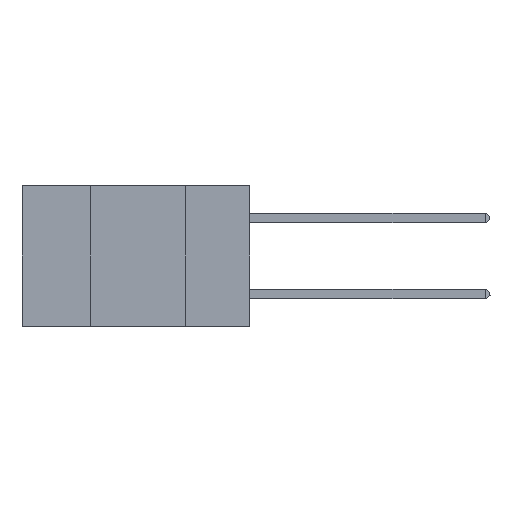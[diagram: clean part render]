
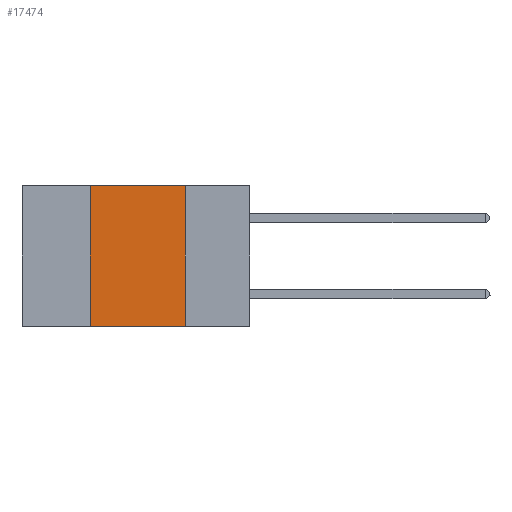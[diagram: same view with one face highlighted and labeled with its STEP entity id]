
A CAD part, left-side view. The second image highlights one B-rep face of the part: STEP entity #17474.
In plain terms, the highlighted planar face has unit normal (-1, 0, 0).
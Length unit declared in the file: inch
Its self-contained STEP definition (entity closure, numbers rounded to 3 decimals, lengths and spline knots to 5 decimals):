
#2667 = ORIENTED_EDGE ( 'NONE', *, *, #25035, .F. ) ;
#2953 = CARTESIAN_POINT ( 'NONE',  ( 0., 0.42, 0. ) ) ;
#3309 = VERTEX_POINT ( 'NONE', #36979 ) ;
#3796 = VERTEX_POINT ( 'NONE', #10225 ) ;
#4160 = DIRECTION ( 'NONE',  ( 1., 0., 0. ) ) ;
#5300 = CARTESIAN_POINT ( 'NONE',  ( 0., 0.17, 0. ) ) ;
#6634 = CARTESIAN_POINT ( 'NONE',  ( 0., 0.42, 0. ) ) ;
#7530 = LINE ( 'NONE', #21985, #16417 ) ;
#8354 = FACE_OUTER_BOUND ( 'NONE', #35504, .T. ) ;
#10193 = LINE ( 'NONE', #6634, #42142 ) ;
#10225 = CARTESIAN_POINT ( 'NONE',  ( 0., 0.42, -0.37 ) ) ;
#12414 = LINE ( 'NONE', #38292, #42146 ) ;
#14400 = PLANE ( 'NONE',  #19005 ) ;
#16417 = VECTOR ( 'NONE', #25111, 39.37008 ) ;
#17474 = ADVANCED_FACE ( 'NONE', ( #8354 ), #14400, .F. ) ;
#17941 = DIRECTION ( 'NONE',  ( 0., 0., -1. ) ) ;
#19005 = AXIS2_PLACEMENT_3D ( 'NONE', #28399, #4160, #17941 ) ;
#20297 = DIRECTION ( 'NONE',  ( 0., 0., -1. ) ) ;
#21507 = VERTEX_POINT ( 'NONE', #2953 ) ;
#21985 = CARTESIAN_POINT ( 'NONE',  ( 0., 0.6, -0.37 ) ) ;
#22859 = DIRECTION ( 'NONE',  ( 0., -1., 0. ) ) ;
#25035 = EDGE_CURVE ( 'NONE', #21507, #41873, #12414, .T. ) ;
#25111 = DIRECTION ( 'NONE',  ( 0., -1., 0. ) ) ;
#27148 = EDGE_CURVE ( 'NONE', #3796, #21507, #10193, .T. ) ;
#28399 = CARTESIAN_POINT ( 'NONE',  ( 0., 0.6, 0. ) ) ;
#30310 = CARTESIAN_POINT ( 'NONE',  ( 0., 0.17, 0. ) ) ;
#34224 = EDGE_CURVE ( 'NONE', #3796, #3309, #7530, .T. ) ;
#34429 = DIRECTION ( 'NONE',  ( 0., 0., 1. ) ) ;
#35362 = EDGE_CURVE ( 'NONE', #41873, #3309, #40548, .T. ) ;
#35504 = EDGE_LOOP ( 'NONE', ( #41393, #2667, #39199, #42919 ) ) ;
#36979 = CARTESIAN_POINT ( 'NONE',  ( 0., 0.17, -0.37 ) ) ;
#38292 = CARTESIAN_POINT ( 'NONE',  ( 0., 0.6, 0. ) ) ;
#39199 = ORIENTED_EDGE ( 'NONE', *, *, #27148, .F. ) ;
#39209 = VECTOR ( 'NONE', #20297, 39.37008 ) ;
#40548 = LINE ( 'NONE', #30310, #39209 ) ;
#41393 = ORIENTED_EDGE ( 'NONE', *, *, #35362, .F. ) ;
#41873 = VERTEX_POINT ( 'NONE', #5300 ) ;
#42142 = VECTOR ( 'NONE', #34429, 39.37008 ) ;
#42146 = VECTOR ( 'NONE', #22859, 39.37008 ) ;
#42919 = ORIENTED_EDGE ( 'NONE', *, *, #34224, .T. ) ;
